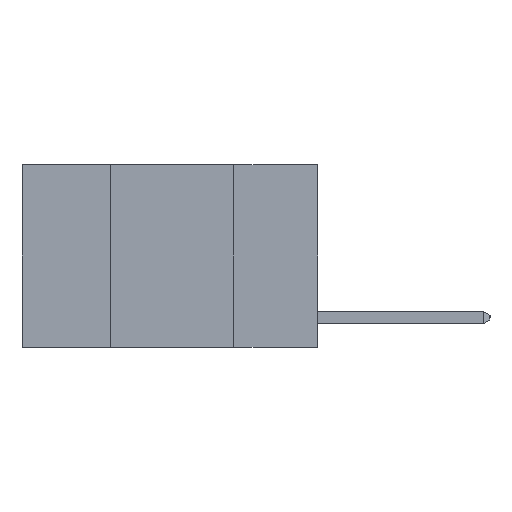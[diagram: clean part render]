
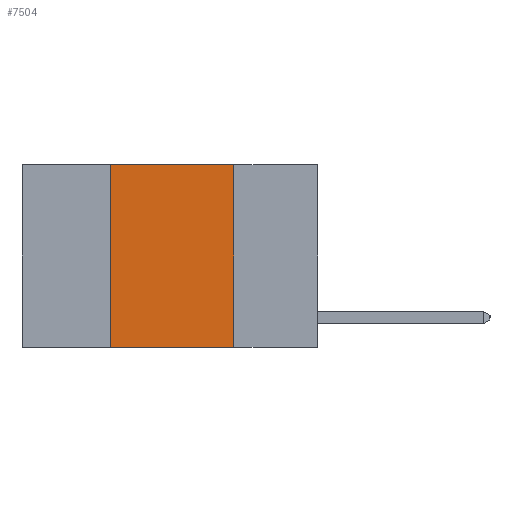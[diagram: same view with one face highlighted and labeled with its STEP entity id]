
A CAD part, left-side view. The second image highlights one B-rep face of the part: STEP entity #7504.
In plain terms, the highlighted planar face has unit normal (-1, 0, 0).
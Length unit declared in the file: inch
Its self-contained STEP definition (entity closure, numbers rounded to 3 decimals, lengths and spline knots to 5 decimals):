
#97 = CARTESIAN_POINT ( 'NONE',  ( 0., 0.42, 0. ) ) ;
#448 = VERTEX_POINT ( 'NONE', #5781 ) ;
#767 = CARTESIAN_POINT ( 'NONE',  ( 0., 0.6, -0.37 ) ) ;
#790 = CARTESIAN_POINT ( 'NONE',  ( 0., 0.6, 0. ) ) ;
#883 = LINE ( 'NONE', #8605, #7533 ) ;
#1025 = VECTOR ( 'NONE', #12393, 39.37008 ) ;
#1884 = VECTOR ( 'NONE', #13640, 39.37008 ) ;
#1978 = VERTEX_POINT ( 'NONE', #97 ) ;
#2353 = ORIENTED_EDGE ( 'NONE', *, *, #14484, .F. ) ;
#3227 = VECTOR ( 'NONE', #13673, 39.37008 ) ;
#3615 = AXIS2_PLACEMENT_3D ( 'NONE', #11066, #6390, #15033 ) ;
#4182 = EDGE_CURVE ( 'NONE', #1978, #11095, #10381, .T. ) ;
#4664 = LINE ( 'NONE', #4941, #1025 ) ;
#4941 = CARTESIAN_POINT ( 'NONE',  ( 0., 0.42, 0. ) ) ;
#5781 = CARTESIAN_POINT ( 'NONE',  ( 0., 0.17, -0.37 ) ) ;
#6390 = DIRECTION ( 'NONE',  ( 1., 0., 0. ) ) ;
#6532 = ORIENTED_EDGE ( 'NONE', *, *, #4182, .F. ) ;
#6583 = CARTESIAN_POINT ( 'NONE',  ( 0., 0.42, -0.37 ) ) ;
#6814 = EDGE_CURVE ( 'NONE', #10147, #448, #10085, .T. ) ;
#7504 = ADVANCED_FACE ( 'NONE', ( #14537 ), #14984, .F. ) ;
#7533 = VECTOR ( 'NONE', #12323, 39.37008 ) ;
#8605 = CARTESIAN_POINT ( 'NONE',  ( 0., 0.17, 0. ) ) ;
#9069 = ORIENTED_EDGE ( 'NONE', *, *, #11461, .F. ) ;
#10085 = LINE ( 'NONE', #767, #3227 ) ;
#10147 = VERTEX_POINT ( 'NONE', #6583 ) ;
#10381 = LINE ( 'NONE', #790, #1884 ) ;
#11066 = CARTESIAN_POINT ( 'NONE',  ( 0., 0.6, 0. ) ) ;
#11095 = VERTEX_POINT ( 'NONE', #12993 ) ;
#11461 = EDGE_CURVE ( 'NONE', #10147, #1978, #4664, .T. ) ;
#12323 = DIRECTION ( 'NONE',  ( 0., 0., -1. ) ) ;
#12393 = DIRECTION ( 'NONE',  ( 0., 0., 1. ) ) ;
#12403 = EDGE_LOOP ( 'NONE', ( #2353, #6532, #9069, #14296 ) ) ;
#12993 = CARTESIAN_POINT ( 'NONE',  ( 0., 0.17, 0. ) ) ;
#13640 = DIRECTION ( 'NONE',  ( 0., -1., 0. ) ) ;
#13673 = DIRECTION ( 'NONE',  ( 0., -1., 0. ) ) ;
#14296 = ORIENTED_EDGE ( 'NONE', *, *, #6814, .T. ) ;
#14484 = EDGE_CURVE ( 'NONE', #11095, #448, #883, .T. ) ;
#14537 = FACE_OUTER_BOUND ( 'NONE', #12403, .T. ) ;
#14984 = PLANE ( 'NONE',  #3615 ) ;
#15033 = DIRECTION ( 'NONE',  ( 0., 0., -1. ) ) ;
